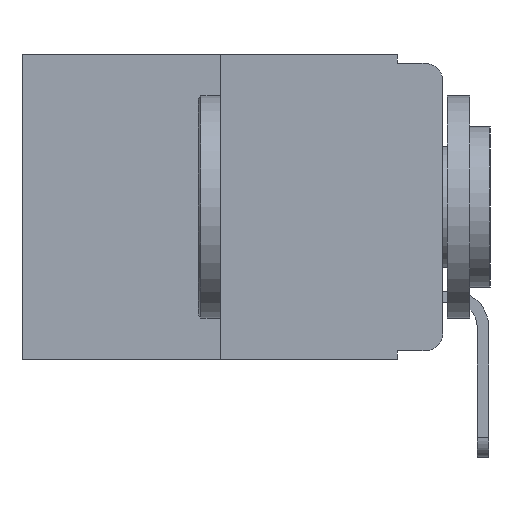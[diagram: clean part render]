
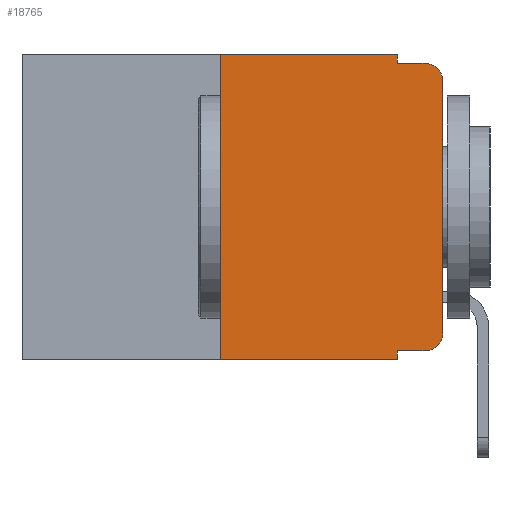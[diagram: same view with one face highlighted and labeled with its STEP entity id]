
A CAD part, left-side view. The second image highlights one B-rep face of the part: STEP entity #18765.
In plain terms, the highlighted planar face has unit normal (-1, 0, 0).
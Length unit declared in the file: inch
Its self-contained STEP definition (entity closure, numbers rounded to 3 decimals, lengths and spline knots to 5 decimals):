
#133 = EDGE_CURVE ( 'NONE', #10348, #3091, #11614, .T. ) ;
#186 = CARTESIAN_POINT ( 'NONE',  ( 0., 0.473, 0. ) ) ;
#252 = DIRECTION ( 'NONE',  ( 0., 0., 1. ) ) ;
#362 = CARTESIAN_POINT ( 'NONE',  ( 0., 0., -0.03 ) ) ;
#728 = ORIENTED_EDGE ( 'NONE', *, *, #133, .T. ) ;
#985 = ORIENTED_EDGE ( 'NONE', *, *, #20695, .F. ) ;
#1100 = VERTEX_POINT ( 'NONE', #4404 ) ;
#1223 = AXIS2_PLACEMENT_3D ( 'NONE', #3750, #18633, #13832 ) ;
#2145 = CARTESIAN_POINT ( 'NONE',  ( 0., 0., -0.313 ) ) ;
#2322 = EDGE_CURVE ( 'NONE', #13638, #10947, #3891, .T. ) ;
#2431 = ORIENTED_EDGE ( 'NONE', *, *, #18696, .F. ) ;
#2676 = CARTESIAN_POINT ( 'NONE',  ( 0., 0.02, -0.313 ) ) ;
#2763 = LINE ( 'NONE', #19077, #5667 ) ;
#2873 = CARTESIAN_POINT ( 'NONE',  ( 0., 0.051, 0. ) ) ;
#3054 = LINE ( 'NONE', #10903, #13022 ) ;
#3091 = VERTEX_POINT ( 'NONE', #14104 ) ;
#3258 = VERTEX_POINT ( 'NONE', #9709 ) ;
#3428 = EDGE_CURVE ( 'NONE', #10947, #10796, #15213, .T. ) ;
#3463 = CARTESIAN_POINT ( 'NONE',  ( 0., 0.02, -0.01 ) ) ;
#3750 = CARTESIAN_POINT ( 'NONE',  ( 0., 0.02, -0.03 ) ) ;
#3891 = LINE ( 'NONE', #7272, #15444 ) ;
#4094 = VERTEX_POINT ( 'NONE', #19293 ) ;
#4160 = DIRECTION ( 'NONE',  ( 0., 0., -1. ) ) ;
#4164 = LINE ( 'NONE', #186, #12545 ) ;
#4358 = DIRECTION ( 'NONE',  ( -1., 0., 0. ) ) ;
#4404 = CARTESIAN_POINT ( 'NONE',  ( 0., 0.02, -0.333 ) ) ;
#4555 = EDGE_CURVE ( 'NONE', #10348, #4094, #9118, .T. ) ;
#5046 = DIRECTION ( 'NONE',  ( 0., -1., 0. ) ) ;
#5653 = EDGE_CURVE ( 'NONE', #3258, #1100, #9159, .T. ) ;
#5667 = VECTOR ( 'NONE', #15769, 39.37008 ) ;
#6368 = EDGE_CURVE ( 'NONE', #3258, #3091, #14254, .T. ) ;
#6835 = DIRECTION ( 'NONE',  ( 1., 0., 0. ) ) ;
#7057 = ORIENTED_EDGE ( 'NONE', *, *, #3428, .T. ) ;
#7272 = CARTESIAN_POINT ( 'NONE',  ( 0., 0., 0. ) ) ;
#7627 = VERTEX_POINT ( 'NONE', #17608 ) ;
#7975 = VECTOR ( 'NONE', #9415, 39.37008 ) ;
#9118 = LINE ( 'NONE', #18969, #16460 ) ;
#9159 = LINE ( 'NONE', #17667, #17814 ) ;
#9354 = CARTESIAN_POINT ( 'NONE',  ( 0., 0.25, -0.343 ) ) ;
#9415 = DIRECTION ( 'NONE',  ( 0., 0., -1. ) ) ;
#9595 = DIRECTION ( 'NONE',  ( 0., -1., 0. ) ) ;
#9709 = CARTESIAN_POINT ( 'NONE',  ( 0., 0.051, -0.333 ) ) ;
#9776 = EDGE_CURVE ( 'NONE', #20581, #7627, #3054, .T. ) ;
#9809 = CARTESIAN_POINT ( 'NONE',  ( 0., 0.473, -0.343 ) ) ;
#10121 = AXIS2_PLACEMENT_3D ( 'NONE', #2676, #4358, #12633 ) ;
#10348 = VERTEX_POINT ( 'NONE', #9354 ) ;
#10796 = VERTEX_POINT ( 'NONE', #3463 ) ;
#10903 = CARTESIAN_POINT ( 'NONE',  ( 0., 0.051, 0. ) ) ;
#10931 = CIRCLE ( 'NONE', #10121, 0.02 ) ;
#10947 = VERTEX_POINT ( 'NONE', #362 ) ;
#11073 = ORIENTED_EDGE ( 'NONE', *, *, #6368, .F. ) ;
#11614 = LINE ( 'NONE', #9809, #16623 ) ;
#11893 = PLANE ( 'NONE',  #14767 ) ;
#11956 = DIRECTION ( 'NONE',  ( 0., -1., 0. ) ) ;
#12060 = ORIENTED_EDGE ( 'NONE', *, *, #9776, .F. ) ;
#12545 = VECTOR ( 'NONE', #11956, 39.37008 ) ;
#12633 = DIRECTION ( 'NONE',  ( 0., 0., -1. ) ) ;
#13022 = VECTOR ( 'NONE', #4160, 39.37008 ) ;
#13584 = DIRECTION ( 'NONE',  ( 0., 0., 1. ) ) ;
#13638 = VERTEX_POINT ( 'NONE', #2145 ) ;
#13832 = DIRECTION ( 'NONE',  ( 0., 0., -1. ) ) ;
#14104 = CARTESIAN_POINT ( 'NONE',  ( 0., 0.051, -0.343 ) ) ;
#14254 = LINE ( 'NONE', #2873, #7975 ) ;
#14736 = ORIENTED_EDGE ( 'NONE', *, *, #2322, .T. ) ;
#14767 = AXIS2_PLACEMENT_3D ( 'NONE', #17016, #6835, #18564 ) ;
#15213 = CIRCLE ( 'NONE', #1223, 0.02 ) ;
#15444 = VECTOR ( 'NONE', #252, 39.37008 ) ;
#15769 = DIRECTION ( 'NONE',  ( 0., -1., 0. ) ) ;
#16236 = FACE_OUTER_BOUND ( 'NONE', #18294, .T. ) ;
#16322 = ORIENTED_EDGE ( 'NONE', *, *, #4555, .F. ) ;
#16460 = VECTOR ( 'NONE', #13584, 39.37008 ) ;
#16623 = VECTOR ( 'NONE', #5046, 39.37008 ) ;
#17016 = CARTESIAN_POINT ( 'NONE',  ( 0., 0.473, 0. ) ) ;
#17023 = CARTESIAN_POINT ( 'NONE',  ( 0., 0.051, 0. ) ) ;
#17501 = EDGE_CURVE ( 'NONE', #1100, #13638, #10931, .T. ) ;
#17608 = CARTESIAN_POINT ( 'NONE',  ( 0., 0.051, -0.01 ) ) ;
#17667 = CARTESIAN_POINT ( 'NONE',  ( 0., 0.051, -0.333 ) ) ;
#17814 = VECTOR ( 'NONE', #9595, 39.37008 ) ;
#18294 = EDGE_LOOP ( 'NONE', ( #14736, #7057, #985, #12060, #2431, #16322, #728, #11073, #18913, #20586 ) ) ;
#18564 = DIRECTION ( 'NONE',  ( 0., 0., -1. ) ) ;
#18633 = DIRECTION ( 'NONE',  ( -1., 0., 0. ) ) ;
#18696 = EDGE_CURVE ( 'NONE', #4094, #20581, #4164, .T. ) ;
#18765 = ADVANCED_FACE ( 'NONE', ( #16236 ), #11893, .F. ) ;
#18913 = ORIENTED_EDGE ( 'NONE', *, *, #5653, .T. ) ;
#18969 = CARTESIAN_POINT ( 'NONE',  ( 0., 0.25, 0. ) ) ;
#19077 = CARTESIAN_POINT ( 'NONE',  ( 0., 0.051, -0.01 ) ) ;
#19293 = CARTESIAN_POINT ( 'NONE',  ( 0., 0.25, 0. ) ) ;
#20581 = VERTEX_POINT ( 'NONE', #17023 ) ;
#20586 = ORIENTED_EDGE ( 'NONE', *, *, #17501, .T. ) ;
#20695 = EDGE_CURVE ( 'NONE', #7627, #10796, #2763, .T. ) ;
